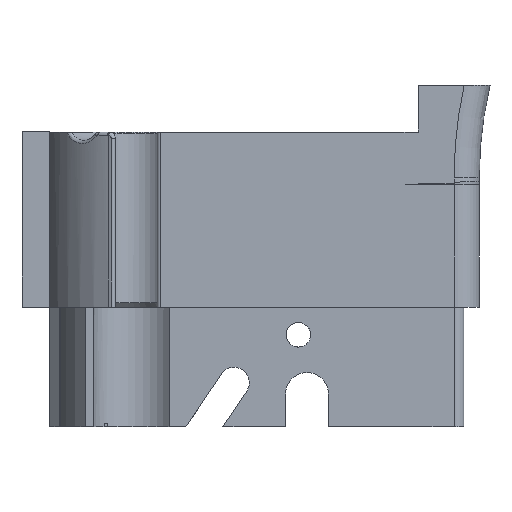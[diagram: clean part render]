
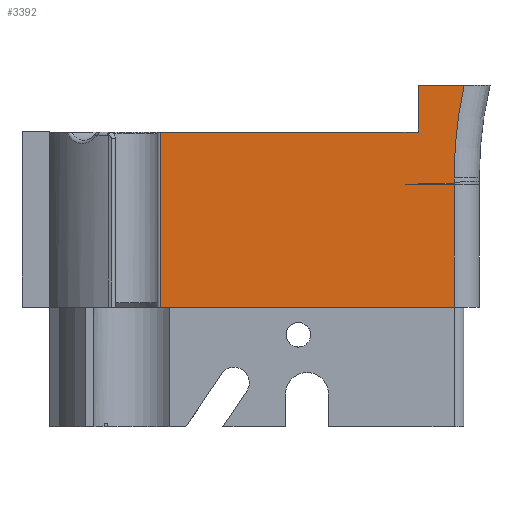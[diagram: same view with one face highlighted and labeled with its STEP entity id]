
A CAD part, left-side view. The second image highlights one B-rep face of the part: STEP entity #3392.
In plain terms, the highlighted planar face has unit normal (-1, 0, 0).
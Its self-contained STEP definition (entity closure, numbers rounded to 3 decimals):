
#95=B_SPLINE_CURVE_WITH_KNOTS('',3,(#5778,#5779,#5780,#5781,#5782),
 .UNSPECIFIED.,.F.,.F.,(4,1,4),(0.,0.77,0.774),
 .UNSPECIFIED.);
#96=B_SPLINE_CURVE_WITH_KNOTS('',3,(#5833,#5834,#5835,#5836,#5837,#5838,
#5839,#5840,#5841,#5842,#5843,#5844),.UNSPECIFIED.,.F.,.F.,(4,1,1,1,1,1,
1,1,1,4),(0.085,0.09,0.095,0.098,
0.101,0.102,0.103,0.103,
0.103,0.103),.UNSPECIFIED.);
#332=FACE_OUTER_BOUND('',#535,.T.);
#535=EDGE_LOOP('',(#2990,#2991,#2992,#2993,#2994,#2995,#2996,#2997,#2998,
#2999,#3000,#3001));
#640=LINE('',#4922,#944);
#658=LINE('',#5008,#962);
#848=LINE('',#5641,#1152);
#849=LINE('',#5726,#1153);
#850=LINE('',#6196,#1154);
#859=LINE('',#6219,#1163);
#862=LINE('',#6271,#1166);
#863=LINE('',#6272,#1167);
#864=LINE('',#6273,#1168);
#944=VECTOR('',#3921,10.);
#962=VECTOR('',#3979,1000.);
#1152=VECTOR('',#4487,10.);
#1153=VECTOR('',#4494,10.);
#1154=VECTOR('',#4517,10.);
#1163=VECTOR('',#4538,10.);
#1166=VECTOR('',#4561,1000.);
#1167=VECTOR('',#4562,1000.);
#1168=VECTOR('',#4563,10.);
#1305=CIRCLE('',#3706,70.448);
#1415=VERTEX_POINT('',#4919);
#1416=VERTEX_POINT('',#4921);
#1441=VERTEX_POINT('',#5005);
#1442=VERTEX_POINT('',#5007);
#1609=VERTEX_POINT('',#5638);
#1610=VERTEX_POINT('',#5640);
#1617=VERTEX_POINT('',#5719);
#1618=VERTEX_POINT('',#5776);
#1619=VERTEX_POINT('',#5831);
#1634=VERTEX_POINT('',#6216);
#1635=VERTEX_POINT('',#6218);
#1638=VERTEX_POINT('',#6267);
#1757=EDGE_CURVE('',#1416,#1415,#640,.T.);
#1793=EDGE_CURVE('',#1442,#1441,#658,.T.);
#2058=EDGE_CURVE('',#1609,#1610,#848,.T.);
#2068=EDGE_CURVE('',#1617,#1609,#849,.T.);
#2071=EDGE_CURVE('',#1618,#1617,#95,.T.);
#2073=EDGE_CURVE('',#1619,#1618,#96,.T.);
#2090=EDGE_CURVE('',#1415,#1610,#850,.T.);
#2099=EDGE_CURVE('',#1635,#1634,#859,.T.);
#2107=EDGE_CURVE('',#1635,#1638,#1305,.T.);
#2109=EDGE_CURVE('',#1638,#1619,#862,.T.);
#2110=EDGE_CURVE('',#1442,#1634,#863,.T.);
#2111=EDGE_CURVE('',#1416,#1441,#864,.T.);
#2990=ORIENTED_EDGE('',*,*,#1757,.T.);
#2991=ORIENTED_EDGE('',*,*,#2090,.T.);
#2992=ORIENTED_EDGE('',*,*,#2058,.F.);
#2993=ORIENTED_EDGE('',*,*,#2068,.F.);
#2994=ORIENTED_EDGE('',*,*,#2071,.F.);
#2995=ORIENTED_EDGE('',*,*,#2073,.F.);
#2996=ORIENTED_EDGE('',*,*,#2109,.F.);
#2997=ORIENTED_EDGE('',*,*,#2107,.F.);
#2998=ORIENTED_EDGE('',*,*,#2099,.T.);
#2999=ORIENTED_EDGE('',*,*,#2110,.F.);
#3000=ORIENTED_EDGE('',*,*,#1793,.T.);
#3001=ORIENTED_EDGE('',*,*,#2111,.F.);
#3241=PLANE('',#3708);
#3392=ADVANCED_FACE('',(#332),#3241,.F.);
#3706=AXIS2_PLACEMENT_3D('',#6268,#4555,#4556);
#3708=AXIS2_PLACEMENT_3D('',#6270,#4559,#4560);
#3921=DIRECTION('',(0.,-1.,0.));
#3979=DIRECTION('',(0.,1.,0.));
#4487=DIRECTION('',(0.,-1.,0.));
#4494=DIRECTION('',(0.,0.,-1.));
#4517=DIRECTION('',(0.,0.,1.));
#4538=DIRECTION('',(0.,1.,0.));
#4555=DIRECTION('center_axis',(-1.,0.,0.));
#4556=DIRECTION('ref_axis',(0.,1.,0.));
#4559=DIRECTION('center_axis',(1.,0.,0.));
#4560=DIRECTION('ref_axis',(0.,1.,0.));
#4561=DIRECTION('',(0.,0.,-1.));
#4562=DIRECTION('',(0.,0.,1.));
#4563=DIRECTION('',(0.,0.,1.));
#4919=CARTESIAN_POINT('',(0.136,-5.842,-7.7));
#4921=CARTESIAN_POINT('',(0.136,42.013,-7.7));
#4922=CARTESIAN_POINT('',(0.136,31.22,-7.7));
#5005=CARTESIAN_POINT('',(0.136,42.013,20.8));
#5007=CARTESIAN_POINT('',(0.136,0.026,20.8));
#5008=CARTESIAN_POINT('',(0.136,30.967,20.8));
#5638=CARTESIAN_POINT('',(0.136,2.058,12.215));
#5640=CARTESIAN_POINT('',(0.136,-5.842,12.215));
#5641=CARTESIAN_POINT('',(0.136,-5.842,12.215));
#5719=CARTESIAN_POINT('',(0.136,2.058,12.3));
#5726=CARTESIAN_POINT('',(0.136,2.058,3.3));
#5776=CARTESIAN_POINT('',(0.136,-5.678,12.471));
#5778=CARTESIAN_POINT('Ctrl Pts',(0.136,-5.678,12.471));
#5779=CARTESIAN_POINT('Ctrl Pts',(0.136,-3.111,12.414));
#5780=CARTESIAN_POINT('Ctrl Pts',(0.136,-0.532,
12.357));
#5781=CARTESIAN_POINT('Ctrl Pts',(0.136,2.046,12.3));
#5782=CARTESIAN_POINT('Ctrl Pts',(0.136,2.058,12.3));
#5831=CARTESIAN_POINT('',(0.136,-5.842,12.547));
#5833=CARTESIAN_POINT('Ctrl Pts',(0.136,-5.842,12.547));
#5834=CARTESIAN_POINT('Ctrl Pts',(0.136,-5.828,12.538));
#5835=CARTESIAN_POINT('Ctrl Pts',(0.136,-5.798,12.519));
#5836=CARTESIAN_POINT('Ctrl Pts',(0.136,-5.76,12.498));
#5837=CARTESIAN_POINT('Ctrl Pts',(0.136,-5.728,12.484));
#5838=CARTESIAN_POINT('Ctrl Pts',(0.136,-5.707,12.477));
#5839=CARTESIAN_POINT('Ctrl Pts',(0.136,-5.693,12.473));
#5840=CARTESIAN_POINT('Ctrl Pts',(0.136,-5.685,12.472));
#5841=CARTESIAN_POINT('Ctrl Pts',(0.136,-5.681,12.471));
#5842=CARTESIAN_POINT('Ctrl Pts',(0.136,-5.679,12.471));
#5843=CARTESIAN_POINT('Ctrl Pts',(0.136,-5.678,12.471));
#5844=CARTESIAN_POINT('Ctrl Pts',(0.136,-5.678,12.471));
#6196=CARTESIAN_POINT('',(0.136,-5.842,-49.7));
#6216=CARTESIAN_POINT('',(0.136,0.026,28.45));
#6218=CARTESIAN_POINT('',(0.136,-7.482,28.45));
#6219=CARTESIAN_POINT('',(0.136,7.731,28.45));
#6267=CARTESIAN_POINT('',(0.136,-5.842,13.335));
#6268=CARTESIAN_POINT('Origin',(0.136,-76.29,13.335));
#6270=CARTESIAN_POINT('Origin',(0.136,33.681,20.8));
#6271=CARTESIAN_POINT('',(0.136,-5.842,20.8));
#6272=CARTESIAN_POINT('',(0.136,0.026,20.8));
#6273=CARTESIAN_POINT('',(0.136,42.013,26.947));
